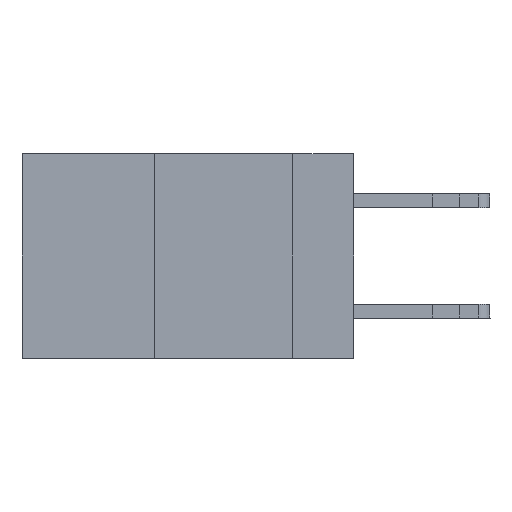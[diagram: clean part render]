
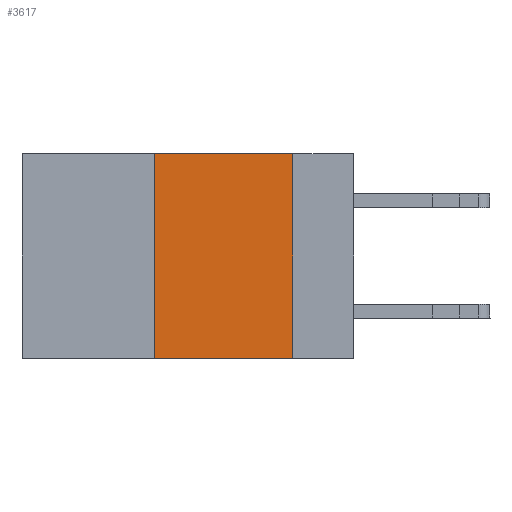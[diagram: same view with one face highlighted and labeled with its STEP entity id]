
A CAD part, left-side view. The second image highlights one B-rep face of the part: STEP entity #3617.
In plain terms, the highlighted planar face has unit normal (-1, 0, 0).
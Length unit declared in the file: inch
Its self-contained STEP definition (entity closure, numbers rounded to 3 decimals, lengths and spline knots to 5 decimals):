
#27 = EDGE_LOOP ( 'NONE', ( #3986, #2403, #3105, #2069 ) ) ;
#479 = DIRECTION ( 'NONE',  ( 0., 0., 1. ) ) ;
#491 = VERTEX_POINT ( 'NONE', #1327 ) ;
#610 = CARTESIAN_POINT ( 'NONE',  ( 0., 0.6, 0. ) ) ;
#841 = VERTEX_POINT ( 'NONE', #9232 ) ;
#878 = DIRECTION ( 'NONE',  ( 0., 0., -1. ) ) ;
#1086 = LINE ( 'NONE', #3760, #13738 ) ;
#1327 = CARTESIAN_POINT ( 'NONE',  ( 0., 0.36, -0.37 ) ) ;
#1484 = EDGE_CURVE ( 'NONE', #12953, #13402, #16385, .T. ) ;
#2069 = ORIENTED_EDGE ( 'NONE', *, *, #7463, .T. ) ;
#2403 = ORIENTED_EDGE ( 'NONE', *, *, #2526, .F. ) ;
#2526 = EDGE_CURVE ( 'NONE', #841, #12953, #15368, .T. ) ;
#3105 = ORIENTED_EDGE ( 'NONE', *, *, #11854, .F. ) ;
#3113 = DIRECTION ( 'NONE',  ( 1., 0., 0. ) ) ;
#3617 = ADVANCED_FACE ( 'NONE', ( #15068 ), #21016, .F. ) ;
#3760 = CARTESIAN_POINT ( 'NONE',  ( 0., 0.36, 0. ) ) ;
#3986 = ORIENTED_EDGE ( 'NONE', *, *, #1484, .F. ) ;
#5104 = CARTESIAN_POINT ( 'NONE',  ( 0., 0.11, 0. ) ) ;
#5626 = VECTOR ( 'NONE', #13828, 39.37008 ) ;
#7463 = EDGE_CURVE ( 'NONE', #491, #13402, #10317, .T. ) ;
#7468 = AXIS2_PLACEMENT_3D ( 'NONE', #11345, #3113, #14639 ) ;
#9125 = CARTESIAN_POINT ( 'NONE',  ( 0., 0.11, 0. ) ) ;
#9232 = CARTESIAN_POINT ( 'NONE',  ( 0., 0.36, 0. ) ) ;
#9790 = VECTOR ( 'NONE', #15030, 39.37008 ) ;
#10317 = LINE ( 'NONE', #16618, #9790 ) ;
#11345 = CARTESIAN_POINT ( 'NONE',  ( 0., 0.6, 0. ) ) ;
#11854 = EDGE_CURVE ( 'NONE', #491, #841, #1086, .T. ) ;
#12098 = VECTOR ( 'NONE', #878, 39.37008 ) ;
#12612 = CARTESIAN_POINT ( 'NONE',  ( 0., 0.11, -0.37 ) ) ;
#12953 = VERTEX_POINT ( 'NONE', #5104 ) ;
#13402 = VERTEX_POINT ( 'NONE', #12612 ) ;
#13738 = VECTOR ( 'NONE', #479, 39.37008 ) ;
#13828 = DIRECTION ( 'NONE',  ( 0., -1., 0. ) ) ;
#14639 = DIRECTION ( 'NONE',  ( 0., 0., -1. ) ) ;
#15030 = DIRECTION ( 'NONE',  ( 0., -1., 0. ) ) ;
#15068 = FACE_OUTER_BOUND ( 'NONE', #27, .T. ) ;
#15368 = LINE ( 'NONE', #610, #5626 ) ;
#16385 = LINE ( 'NONE', #9125, #12098 ) ;
#16618 = CARTESIAN_POINT ( 'NONE',  ( 0., 0.6, -0.37 ) ) ;
#21016 = PLANE ( 'NONE',  #7468 ) ;
